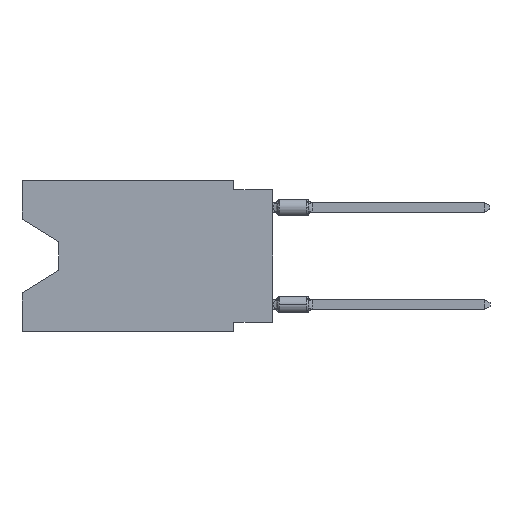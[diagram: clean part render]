
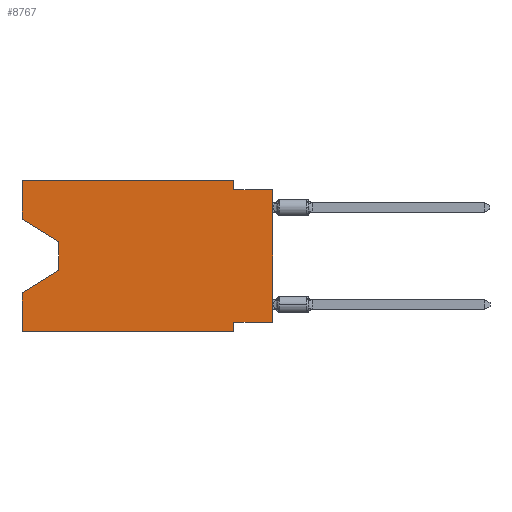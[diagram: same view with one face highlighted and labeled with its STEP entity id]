
A CAD part, left-side view. The second image highlights one B-rep face of the part: STEP entity #8767.
In plain terms, the highlighted planar face has unit normal (-1, 0, 0).
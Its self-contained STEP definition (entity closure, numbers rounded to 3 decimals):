
#205 = AXIS2_PLACEMENT_3D ( 'NONE', #22965, #9906, #9774 ) ;
#295 = VERTEX_POINT ( 'NONE', #17898 ) ;
#327 = LINE ( 'NONE', #7409, #20999 ) ;
#796 = CARTESIAN_POINT ( 'NONE',  ( 0., 13.97, -5.893 ) ) ;
#836 = EDGE_CURVE ( 'NONE', #12006, #3799, #10248, .T. ) ;
#985 = ORIENTED_EDGE ( 'NONE', *, *, #836, .T. ) ;
#994 = VERTEX_POINT ( 'NONE', #18075 ) ;
#1727 = EDGE_CURVE ( 'NONE', #16088, #14110, #19748, .T. ) ;
#1734 = VECTOR ( 'NONE', #26062, 1000. ) ;
#1890 = EDGE_CURVE ( 'NONE', #22564, #994, #327, .T. ) ;
#2087 = VERTEX_POINT ( 'NONE', #23723 ) ;
#3522 = CARTESIAN_POINT ( 'NONE',  ( 0., 16.383, -9.906 ) ) ;
#3559 = VECTOR ( 'NONE', #9248, 1000. ) ;
#3581 = PLANE ( 'NONE',  #205 ) ;
#3799 = VERTEX_POINT ( 'NONE', #5503 ) ;
#4563 = CARTESIAN_POINT ( 'NONE',  ( 0., 2.54, -9.271 ) ) ;
#5028 = DIRECTION ( 'NONE',  ( 0., 0., 1. ) ) ;
#5503 = CARTESIAN_POINT ( 'NONE',  ( 0., 13.97, -4.013 ) ) ;
#5867 = ORIENTED_EDGE ( 'NONE', *, *, #1727, .F. ) ;
#6702 = ORIENTED_EDGE ( 'NONE', *, *, #7025, .F. ) ;
#6923 = VECTOR ( 'NONE', #25577, 1000. ) ;
#7025 = EDGE_CURVE ( 'NONE', #994, #11916, #20725, .T. ) ;
#7409 = CARTESIAN_POINT ( 'NONE',  ( 0., 16.383, 0. ) ) ;
#8137 = VECTOR ( 'NONE', #12407, 1000. ) ;
#8558 = VECTOR ( 'NONE', #20870, 1000. ) ;
#8749 = DIRECTION ( 'NONE',  ( 0., 0., 1. ) ) ;
#8767 = ADVANCED_FACE ( 'NONE', ( #27142 ), #3581, .F. ) ;
#9248 = DIRECTION ( 'NONE',  ( 0., 0., -1. ) ) ;
#9774 = DIRECTION ( 'NONE',  ( 0., 0., -1. ) ) ;
#9906 = DIRECTION ( 'NONE',  ( 1., 0., 0. ) ) ;
#10164 = VECTOR ( 'NONE', #8749, 1000. ) ;
#10248 = LINE ( 'NONE', #15117, #8137 ) ;
#10423 = CARTESIAN_POINT ( 'NONE',  ( 0., 0., -9.271 ) ) ;
#10512 = CARTESIAN_POINT ( 'NONE',  ( 0., 16.383, -9.906 ) ) ;
#10668 = EDGE_CURVE ( 'NONE', #16088, #16772, #12116, .T. ) ;
#11226 = CARTESIAN_POINT ( 'NONE',  ( 0., 16.383, 0. ) ) ;
#11775 = LINE ( 'NONE', #22674, #19411 ) ;
#11916 = VERTEX_POINT ( 'NONE', #17828 ) ;
#12006 = VERTEX_POINT ( 'NONE', #26021 ) ;
#12023 = DIRECTION ( 'NONE',  ( 0., 0.855, -0.519 ) ) ;
#12116 = LINE ( 'NONE', #18868, #8558 ) ;
#12346 = ORIENTED_EDGE ( 'NONE', *, *, #22475, .T. ) ;
#12407 = DIRECTION ( 'NONE',  ( 0., -0.855, -0.519 ) ) ;
#12535 = ORIENTED_EDGE ( 'NONE', *, *, #10668, .T. ) ;
#13868 = EDGE_CURVE ( 'NONE', #11916, #16772, #11775, .T. ) ;
#14036 = CARTESIAN_POINT ( 'NONE',  ( 0., 0., -0.635 ) ) ;
#14110 = VERTEX_POINT ( 'NONE', #4563 ) ;
#15117 = CARTESIAN_POINT ( 'NONE',  ( 0., 16.383, -2.546 ) ) ;
#15230 = LINE ( 'NONE', #21830, #20214 ) ;
#16088 = VERTEX_POINT ( 'NONE', #18989 ) ;
#16772 = VERTEX_POINT ( 'NONE', #14036 ) ;
#17190 = ORIENTED_EDGE ( 'NONE', *, *, #1890, .F. ) ;
#17694 = EDGE_CURVE ( 'NONE', #14110, #295, #20859, .T. ) ;
#17706 = ORIENTED_EDGE ( 'NONE', *, *, #22051, .T. ) ;
#17804 = DIRECTION ( 'NONE',  ( 0., 0., -1. ) ) ;
#17828 = CARTESIAN_POINT ( 'NONE',  ( 0., 2.54, -0.635 ) ) ;
#17898 = CARTESIAN_POINT ( 'NONE',  ( 0., 2.54, -9.906 ) ) ;
#17918 = LINE ( 'NONE', #19650, #10164 ) ;
#18064 = VERTEX_POINT ( 'NONE', #27376 ) ;
#18075 = CARTESIAN_POINT ( 'NONE',  ( 0., 2.54, 0. ) ) ;
#18238 = LINE ( 'NONE', #11226, #22821 ) ;
#18567 = ORIENTED_EDGE ( 'NONE', *, *, #17694, .F. ) ;
#18854 = DIRECTION ( 'NONE',  ( 0., 0., -1. ) ) ;
#18868 = CARTESIAN_POINT ( 'NONE',  ( 0., 0., 0. ) ) ;
#18989 = CARTESIAN_POINT ( 'NONE',  ( 0., 0., -9.271 ) ) ;
#19288 = EDGE_CURVE ( 'NONE', #12006, #22564, #18238, .T. ) ;
#19411 = VECTOR ( 'NONE', #23089, 1000. ) ;
#19650 = CARTESIAN_POINT ( 'NONE',  ( 0., 16.383, 0. ) ) ;
#19748 = LINE ( 'NONE', #10423, #1734 ) ;
#20002 = VECTOR ( 'NONE', #18854, 1000. ) ;
#20214 = VECTOR ( 'NONE', #17804, 1000. ) ;
#20725 = LINE ( 'NONE', #22572, #3559 ) ;
#20859 = LINE ( 'NONE', #25304, #20002 ) ;
#20870 = DIRECTION ( 'NONE',  ( 0., 0., 1. ) ) ;
#20999 = VECTOR ( 'NONE', #26905, 1000. ) ;
#21273 = CARTESIAN_POINT ( 'NONE',  ( 0., 16.383, 0. ) ) ;
#21830 = CARTESIAN_POINT ( 'NONE',  ( 0., 13.97, -4.013 ) ) ;
#21874 = ORIENTED_EDGE ( 'NONE', *, *, #13868, .F. ) ;
#22051 = EDGE_CURVE ( 'NONE', #2087, #18064, #22345, .T. ) ;
#22345 = LINE ( 'NONE', #796, #25689 ) ;
#22475 = EDGE_CURVE ( 'NONE', #24222, #295, #25997, .T. ) ;
#22564 = VERTEX_POINT ( 'NONE', #21273 ) ;
#22572 = CARTESIAN_POINT ( 'NONE',  ( 0., 2.54, 0. ) ) ;
#22651 = EDGE_CURVE ( 'NONE', #3799, #2087, #15230, .T. ) ;
#22674 = CARTESIAN_POINT ( 'NONE',  ( 0., 0., -0.635 ) ) ;
#22821 = VECTOR ( 'NONE', #5028, 1000. ) ;
#22965 = CARTESIAN_POINT ( 'NONE',  ( 0., 16.383, 0. ) ) ;
#23089 = DIRECTION ( 'NONE',  ( 0., -1., 0. ) ) ;
#23499 = EDGE_LOOP ( 'NONE', ( #985, #25822, #17706, #25536, #12346, #18567, #5867, #12535, #21874, #6702, #17190, #26982 ) ) ;
#23723 = CARTESIAN_POINT ( 'NONE',  ( 0., 13.97, -5.893 ) ) ;
#24222 = VERTEX_POINT ( 'NONE', #3522 ) ;
#25304 = CARTESIAN_POINT ( 'NONE',  ( 0., 2.54, -9.906 ) ) ;
#25536 = ORIENTED_EDGE ( 'NONE', *, *, #26908, .F. ) ;
#25577 = DIRECTION ( 'NONE',  ( 0., -1., 0. ) ) ;
#25689 = VECTOR ( 'NONE', #12023, 1000. ) ;
#25822 = ORIENTED_EDGE ( 'NONE', *, *, #22651, .T. ) ;
#25997 = LINE ( 'NONE', #10512, #6923 ) ;
#26021 = CARTESIAN_POINT ( 'NONE',  ( 0., 16.383, -2.546 ) ) ;
#26062 = DIRECTION ( 'NONE',  ( 0., 1., 0. ) ) ;
#26905 = DIRECTION ( 'NONE',  ( 0., -1., 0. ) ) ;
#26908 = EDGE_CURVE ( 'NONE', #24222, #18064, #17918, .T. ) ;
#26982 = ORIENTED_EDGE ( 'NONE', *, *, #19288, .F. ) ;
#27142 = FACE_OUTER_BOUND ( 'NONE', #23499, .T. ) ;
#27376 = CARTESIAN_POINT ( 'NONE',  ( 0., 16.383, -7.36 ) ) ;
